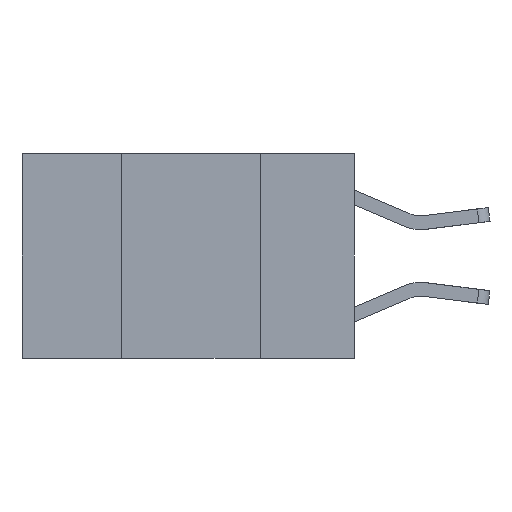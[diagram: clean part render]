
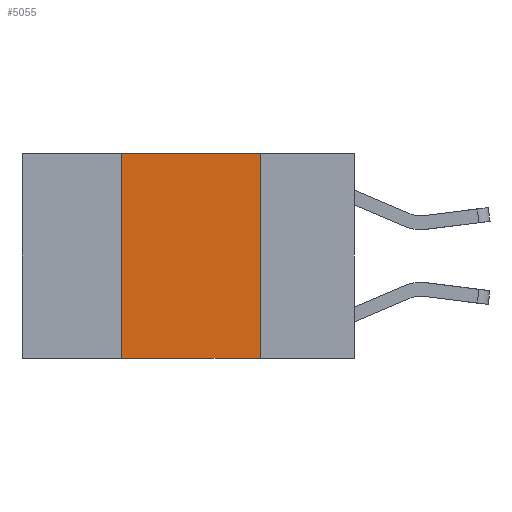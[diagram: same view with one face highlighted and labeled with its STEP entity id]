
A CAD part, left-side view. The second image highlights one B-rep face of the part: STEP entity #5055.
In plain terms, the highlighted planar face has unit normal (-1, 0, 0).
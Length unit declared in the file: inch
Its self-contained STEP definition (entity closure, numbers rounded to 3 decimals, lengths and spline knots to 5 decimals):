
#184 = ORIENTED_EDGE ( 'NONE', *, *, #7491, .T. ) ;
#380 = ORIENTED_EDGE ( 'NONE', *, *, #7356, .F. ) ;
#406 = DIRECTION ( 'NONE',  ( 1., 0., 0. ) ) ;
#753 = VERTEX_POINT ( 'NONE', #3579 ) ;
#1393 = CARTESIAN_POINT ( 'NONE',  ( 0., 0.42, -0.37 ) ) ;
#1521 = CARTESIAN_POINT ( 'NONE',  ( 0., 0.42, 0. ) ) ;
#1860 = EDGE_LOOP ( 'NONE', ( #7408, #10343, #380, #184 ) ) ;
#1948 = VECTOR ( 'NONE', #6719, 39.37008 ) ;
#2359 = DIRECTION ( 'NONE',  ( 0., 0., 1. ) ) ;
#2745 = DIRECTION ( 'NONE',  ( 0., 0., -1. ) ) ;
#3173 = CARTESIAN_POINT ( 'NONE',  ( 0., 0.17, 0. ) ) ;
#3292 = VERTEX_POINT ( 'NONE', #1393 ) ;
#3579 = CARTESIAN_POINT ( 'NONE',  ( 0., 0.17, -0.37 ) ) ;
#4129 = CARTESIAN_POINT ( 'NONE',  ( 0., 0.6, 0. ) ) ;
#4454 = CARTESIAN_POINT ( 'NONE',  ( 0., 0.17, 0. ) ) ;
#5055 = ADVANCED_FACE ( 'NONE', ( #10055 ), #7155, .F. ) ;
#5188 = LINE ( 'NONE', #4129, #9662 ) ;
#5485 = LINE ( 'NONE', #4454, #10216 ) ;
#5528 = LINE ( 'NONE', #1521, #9745 ) ;
#6346 = DIRECTION ( 'NONE',  ( 0., 0., -1. ) ) ;
#6719 = DIRECTION ( 'NONE',  ( 0., -1., 0. ) ) ;
#7078 = VERTEX_POINT ( 'NONE', #9634 ) ;
#7155 = PLANE ( 'NONE',  #10743 ) ;
#7356 = EDGE_CURVE ( 'NONE', #3292, #7078, #5528, .T. ) ;
#7408 = ORIENTED_EDGE ( 'NONE', *, *, #8320, .F. ) ;
#7491 = EDGE_CURVE ( 'NONE', #3292, #753, #10902, .T. ) ;
#8320 = EDGE_CURVE ( 'NONE', #10030, #753, #5485, .T. ) ;
#8321 = DIRECTION ( 'NONE',  ( 0., -1., 0. ) ) ;
#8860 = CARTESIAN_POINT ( 'NONE',  ( 0., 0.6, 0. ) ) ;
#9226 = CARTESIAN_POINT ( 'NONE',  ( 0., 0.6, -0.37 ) ) ;
#9634 = CARTESIAN_POINT ( 'NONE',  ( 0., 0.42, 0. ) ) ;
#9662 = VECTOR ( 'NONE', #8321, 39.37008 ) ;
#9745 = VECTOR ( 'NONE', #2359, 39.37008 ) ;
#10030 = VERTEX_POINT ( 'NONE', #3173 ) ;
#10055 = FACE_OUTER_BOUND ( 'NONE', #1860, .T. ) ;
#10126 = EDGE_CURVE ( 'NONE', #7078, #10030, #5188, .T. ) ;
#10216 = VECTOR ( 'NONE', #2745, 39.37008 ) ;
#10343 = ORIENTED_EDGE ( 'NONE', *, *, #10126, .F. ) ;
#10743 = AXIS2_PLACEMENT_3D ( 'NONE', #8860, #406, #6346 ) ;
#10902 = LINE ( 'NONE', #9226, #1948 ) ;
